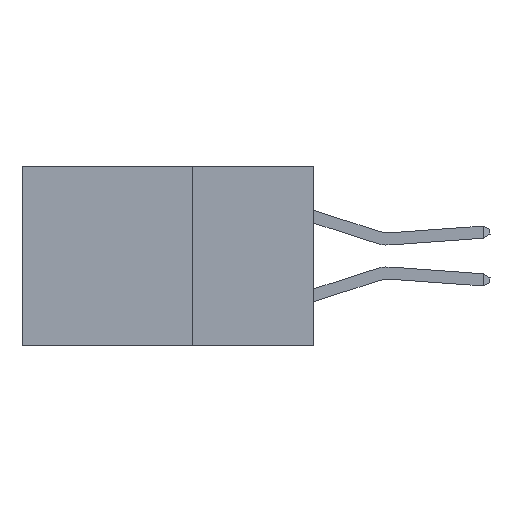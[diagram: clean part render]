
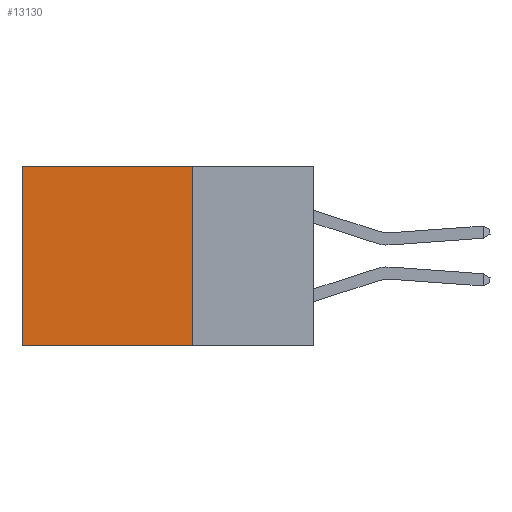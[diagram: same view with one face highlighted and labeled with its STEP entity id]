
A CAD part, left-side view. The second image highlights one B-rep face of the part: STEP entity #13130.
In plain terms, the highlighted planar face has unit normal (-1, 0, 0).
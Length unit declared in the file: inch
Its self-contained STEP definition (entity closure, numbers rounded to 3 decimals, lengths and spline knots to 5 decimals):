
#172 = ORIENTED_EDGE ( 'NONE', *, *, #6673, .T. ) ;
#475 = ORIENTED_EDGE ( 'NONE', *, *, #9043, .F. ) ;
#1838 = DIRECTION ( 'NONE',  ( 0., 0., -1. ) ) ;
#2312 = CARTESIAN_POINT ( 'NONE',  ( 0.2875, 0.6, 0. ) ) ;
#2562 = CARTESIAN_POINT ( 'NONE',  ( 0.2875, 0.25, 0. ) ) ;
#3303 = VECTOR ( 'NONE', #13589, 39.37008 ) ;
#4323 = LINE ( 'NONE', #5113, #9250 ) ;
#4368 = EDGE_CURVE ( 'NONE', #18826, #16975, #7625, .T. ) ;
#4703 = CARTESIAN_POINT ( 'NONE',  ( 0.2875, 0.6, -0.37 ) ) ;
#4948 = LINE ( 'NONE', #2562, #18844 ) ;
#5113 = CARTESIAN_POINT ( 'NONE',  ( 0.2875, 0.25, 0. ) ) ;
#6673 = EDGE_CURVE ( 'NONE', #13183, #16786, #4323, .T. ) ;
#6712 = EDGE_CURVE ( 'NONE', #16786, #16975, #18797, .T. ) ;
#7078 = CARTESIAN_POINT ( 'NONE',  ( 0.2875, 0.6, 0. ) ) ;
#7625 = LINE ( 'NONE', #13616, #3303 ) ;
#9043 = EDGE_CURVE ( 'NONE', #13183, #18826, #4948, .T. ) ;
#9250 = VECTOR ( 'NONE', #14261, 39.37008 ) ;
#12143 = ORIENTED_EDGE ( 'NONE', *, *, #6712, .T. ) ;
#12605 = AXIS2_PLACEMENT_3D ( 'NONE', #19908, #12837, #1838 ) ;
#12837 = DIRECTION ( 'NONE',  ( 1., 0., 0. ) ) ;
#13130 = ADVANCED_FACE ( 'NONE', ( #15083 ), #13226, .F. ) ;
#13183 = VERTEX_POINT ( 'NONE', #21776 ) ;
#13226 = PLANE ( 'NONE',  #12605 ) ;
#13532 = DIRECTION ( 'NONE',  ( 0., 0., -1. ) ) ;
#13589 = DIRECTION ( 'NONE',  ( 0., 1., 0. ) ) ;
#13616 = CARTESIAN_POINT ( 'NONE',  ( 0.2875, 0.25, -0.37 ) ) ;
#14261 = DIRECTION ( 'NONE',  ( 0., 1., 0. ) ) ;
#14336 = DIRECTION ( 'NONE',  ( 0., 0., -1. ) ) ;
#15083 = FACE_OUTER_BOUND ( 'NONE', #18408, .T. ) ;
#16596 = ORIENTED_EDGE ( 'NONE', *, *, #4368, .F. ) ;
#16786 = VERTEX_POINT ( 'NONE', #2312 ) ;
#16975 = VERTEX_POINT ( 'NONE', #4703 ) ;
#17724 = VECTOR ( 'NONE', #14336, 39.37008 ) ;
#18408 = EDGE_LOOP ( 'NONE', ( #12143, #16596, #475, #172 ) ) ;
#18797 = LINE ( 'NONE', #7078, #17724 ) ;
#18826 = VERTEX_POINT ( 'NONE', #22597 ) ;
#18844 = VECTOR ( 'NONE', #13532, 39.37008 ) ;
#19908 = CARTESIAN_POINT ( 'NONE',  ( 0.2875, 0.25, 0. ) ) ;
#21776 = CARTESIAN_POINT ( 'NONE',  ( 0.2875, 0.25, 0. ) ) ;
#22597 = CARTESIAN_POINT ( 'NONE',  ( 0.2875, 0.25, -0.37 ) ) ;
